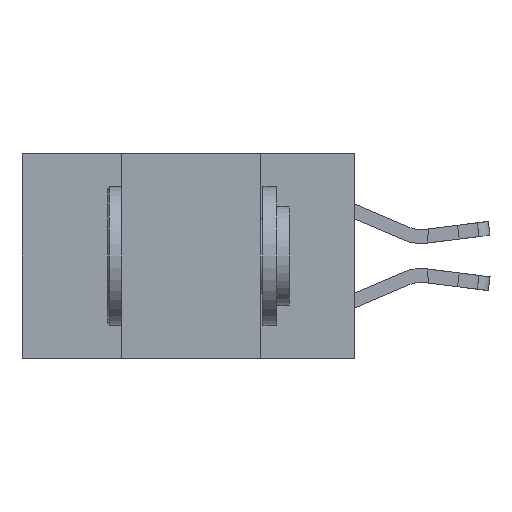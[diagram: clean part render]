
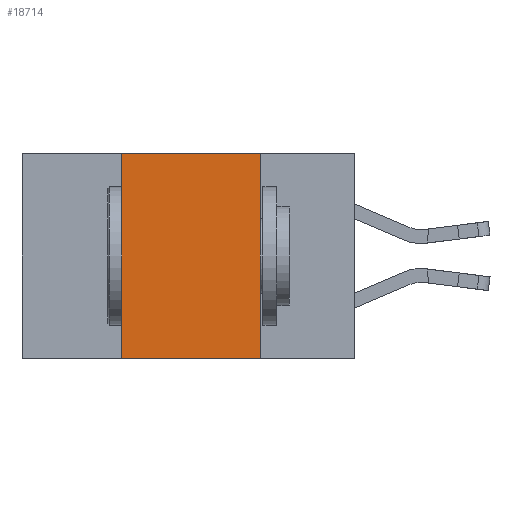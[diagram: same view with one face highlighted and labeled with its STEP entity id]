
A CAD part, left-side view. The second image highlights one B-rep face of the part: STEP entity #18714.
In plain terms, the highlighted planar face has unit normal (-1, 0, 0).
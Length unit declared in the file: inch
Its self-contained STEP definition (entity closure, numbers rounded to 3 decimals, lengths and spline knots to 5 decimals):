
#54 = ORIENTED_EDGE ( 'NONE', *, *, #23680, .F. ) ;
#313 = EDGE_LOOP ( 'NONE', ( #3286, #6970, #54, #18241 ) ) ;
#1985 = CARTESIAN_POINT ( 'NONE',  ( 0., 0.17, -0.37 ) ) ;
#2174 = CARTESIAN_POINT ( 'NONE',  ( 0., 0.42, -0.37 ) ) ;
#3148 = CARTESIAN_POINT ( 'NONE',  ( 0., 0.17, 0. ) ) ;
#3286 = ORIENTED_EDGE ( 'NONE', *, *, #24175, .F. ) ;
#3581 = LINE ( 'NONE', #8999, #22400 ) ;
#4746 = CARTESIAN_POINT ( 'NONE',  ( 0., 0.42, 0. ) ) ;
#4824 = VECTOR ( 'NONE', #15407, 39.37008 ) ;
#4870 = DIRECTION ( 'NONE',  ( 0., -1., 0. ) ) ;
#5288 = FACE_OUTER_BOUND ( 'NONE', #313, .T. ) ;
#6663 = PLANE ( 'NONE',  #9099 ) ;
#6970 = ORIENTED_EDGE ( 'NONE', *, *, #11402, .F. ) ;
#7986 = VERTEX_POINT ( 'NONE', #4746 ) ;
#8412 = LINE ( 'NONE', #26919, #19025 ) ;
#8795 = CARTESIAN_POINT ( 'NONE',  ( 0., 0.6, 0. ) ) ;
#8999 = CARTESIAN_POINT ( 'NONE',  ( 0., 0.6, 0. ) ) ;
#9099 = AXIS2_PLACEMENT_3D ( 'NONE', #8795, #14741, #19181 ) ;
#9682 = VERTEX_POINT ( 'NONE', #2174 ) ;
#10440 = LINE ( 'NONE', #13270, #4824 ) ;
#11184 = VERTEX_POINT ( 'NONE', #3148 ) ;
#11402 = EDGE_CURVE ( 'NONE', #7986, #11184, #3581, .T. ) ;
#13270 = CARTESIAN_POINT ( 'NONE',  ( 0., 0.6, -0.37 ) ) ;
#13498 = EDGE_CURVE ( 'NONE', #9682, #26977, #10440, .T. ) ;
#13899 = DIRECTION ( 'NONE',  ( 0., 0., 1. ) ) ;
#14097 = DIRECTION ( 'NONE',  ( 0., 0., -1. ) ) ;
#14164 = CARTESIAN_POINT ( 'NONE',  ( 0., 0.42, 0. ) ) ;
#14741 = DIRECTION ( 'NONE',  ( 1., 0., 0. ) ) ;
#14748 = LINE ( 'NONE', #14164, #20043 ) ;
#15407 = DIRECTION ( 'NONE',  ( 0., -1., 0. ) ) ;
#18241 = ORIENTED_EDGE ( 'NONE', *, *, #13498, .T. ) ;
#18714 = ADVANCED_FACE ( 'NONE', ( #5288 ), #6663, .F. ) ;
#19025 = VECTOR ( 'NONE', #14097, 39.37008 ) ;
#19181 = DIRECTION ( 'NONE',  ( 0., 0., -1. ) ) ;
#20043 = VECTOR ( 'NONE', #13899, 39.37008 ) ;
#22400 = VECTOR ( 'NONE', #4870, 39.37008 ) ;
#23680 = EDGE_CURVE ( 'NONE', #9682, #7986, #14748, .T. ) ;
#24175 = EDGE_CURVE ( 'NONE', #11184, #26977, #8412, .T. ) ;
#26919 = CARTESIAN_POINT ( 'NONE',  ( 0., 0.17, 0. ) ) ;
#26977 = VERTEX_POINT ( 'NONE', #1985 ) ;
